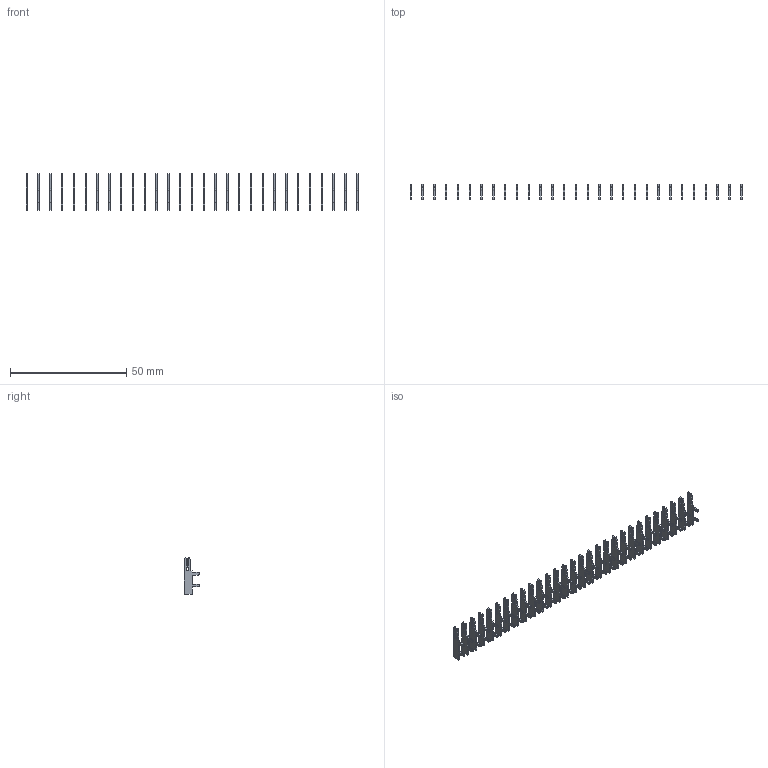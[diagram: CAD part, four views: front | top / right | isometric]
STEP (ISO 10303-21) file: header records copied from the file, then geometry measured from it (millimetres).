
FILE_DESCRIPTION (( 'STEP AP203' ), '1' );
FILE_NAME ('105-029-202-200.STEP', '2020-04-07T23:23:02', ( '' ), ( '' ), 'SwSTEP 2.0', 'SolidWorks 2016', '' );
FILE_SCHEMA (( 'CONFIG_CONTROL_DESIGN' ));
Length unit declared in the file: inch
Products named in the file (2): 105-029-202-200; 100-290-001_100-290-202
Assembly tree (29 placements, depth 2):
  105-029-202-200
    100-290-001_100-290-202  x29
Bounding box: 142.84 x 6.53 x 15.88 mm (x, y, z)
Volume: 921.4 mm3; surface area: 4097.7 mm2
Topology: 29 solids, 29 shells, 870 faces, 2436 edges, 1624 vertices
Faces by surface type: plane 667, cylinder 203
Entity records: 2058 total; most frequent: DIRECTION 218, CARTESIAN_POINT 214, ORIENTED_EDGE 168, EDGE_CURVE 84, AXIS2_PLACEMENT_3D 76, LOCAL_TIME 68, DATE_AND_TIME 68, CALENDAR_DATE 68
